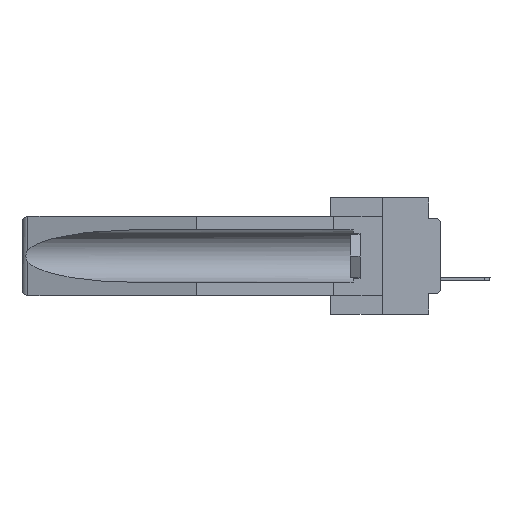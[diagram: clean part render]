
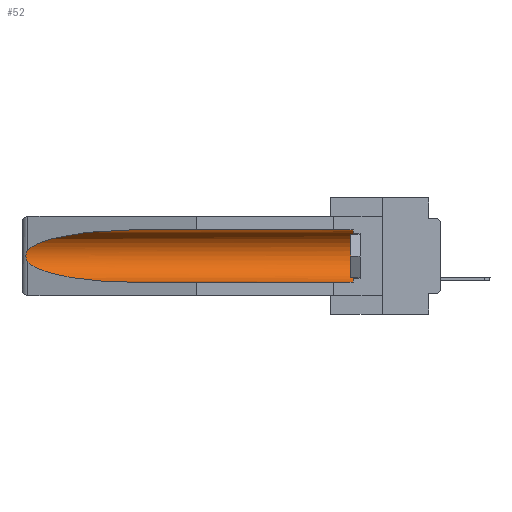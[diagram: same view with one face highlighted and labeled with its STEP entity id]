
A CAD part, left-side view. The second image highlights one B-rep face of the part: STEP entity #52.
In plain terms, the highlighted cylindrical face has radius 2.857 mm (diameter 5.715 mm), a partial arc.
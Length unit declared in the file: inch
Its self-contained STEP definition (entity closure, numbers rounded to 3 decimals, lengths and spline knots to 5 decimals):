
#52 = ADVANCED_FACE ( 'NONE', ( #21755 ), #23921, .F. ) ;
#111 = B_SPLINE_CURVE_WITH_KNOTS ( 'NONE', 3,
 ( #18449, #18297, #6467, #27815, #15988, #25214, #16144, #2009, #18753, #25517 ),
 .UNSPECIFIED., .F., .F.,
 ( 4, 2, 2, 2, 4 ),
 ( 0., 0.00029, 0.00058, 0.00087, 0.00117 ),
 .UNSPECIFIED. ) ;
#756 = VECTOR ( 'NONE', #5604, 39.37008 ) ;
#907 = DIRECTION ( 'NONE',  ( 0., 0., 1. ) ) ;
#1017 = LINE ( 'NONE', #10353, #756 ) ;
#1035 = LINE ( 'NONE', #10519, #4008 ) ;
#1042 = EDGE_CURVE ( 'NONE', #15640, #15206, #111, .T. ) ;
#1517 = CARTESIAN_POINT ( 'NONE',  ( 0.155, 1.07973, -0.059 ) ) ;
#2009 = CARTESIAN_POINT ( 'NONE',  ( 0.26655, 1.53094, -0.18657 ) ) ;
#2273 = VERTEX_POINT ( 'NONE', #16155 ) ;
#4008 = VECTOR ( 'NONE', #27600, 39.37008 ) ;
#4174 = EDGE_CURVE ( 'NONE', #28721, #12093, #25974, .T. ) ;
#4538 =( BOUNDED_CURVE ( )  B_SPLINE_CURVE ( 3, ( #1517, #29317, #10863, #10254 ),
 .UNSPECIFIED., .F., .F. ) 
 B_SPLINE_CURVE_WITH_KNOTS ( ( 4, 4 ),
 ( 4.71239, 6.08839 ),
 .UNSPECIFIED. ) 
 CURVE ( )  GEOMETRIC_REPRESENTATION_ITEM ( )  RATIONAL_B_SPLINE_CURVE ( ( 1., 0.848, 0.848, 1. ) ) 
 REPRESENTATION_ITEM ( '' )  );
#5159 = AXIS2_PLACEMENT_3D ( 'NONE', #24554, #22099, #907 ) ;
#5604 = DIRECTION ( 'NONE',  ( 0., 1., 0. ) ) ;
#5646 = EDGE_CURVE ( 'NONE', #12093, #2273, #1017, .T. ) ;
#6467 = CARTESIAN_POINT ( 'NONE',  ( 0.26654, 1.53092, -0.15636 ) ) ;
#7896 = ORIENTED_EDGE ( 'NONE', *, *, #11293, .T. ) ;
#9016 = AXIS2_PLACEMENT_3D ( 'NONE', #21608, #14836, #9902 ) ;
#9123 = ORIENTED_EDGE ( 'NONE', *, *, #5646, .T. ) ;
#9902 = DIRECTION ( 'NONE',  ( 0., 0., 1. ) ) ;
#10254 = CARTESIAN_POINT ( 'NONE',  ( 0.26537, 1.52718, -0.14972 ) ) ;
#10353 = CARTESIAN_POINT ( 'NONE',  ( 0.155, -0.30754, -0.059 ) ) ;
#10519 = CARTESIAN_POINT ( 'NONE',  ( 0.155, -0.30754, -0.284 ) ) ;
#10863 = CARTESIAN_POINT ( 'NONE',  ( 0.25451, 1.48313, -0.09465 ) ) ;
#10957 = CARTESIAN_POINT ( 'NONE',  ( 0.21114, 1.30732, -0.284 ) ) ;
#11293 = EDGE_CURVE ( 'NONE', #15206, #25546, #17063, .T. ) ;
#12093 = VERTEX_POINT ( 'NONE', #14445 ) ;
#12406 = EDGE_CURVE ( 'NONE', #2273, #15640, #4538, .T. ) ;
#12456 = CARTESIAN_POINT ( 'NONE',  ( 0.155, 0.126, -0.284 ) ) ;
#13138 = CARTESIAN_POINT ( 'NONE',  ( 0.25451, 1.48313, -0.24835 ) ) ;
#13657 = ORIENTED_EDGE ( 'NONE', *, *, #14958, .F. ) ;
#14445 = CARTESIAN_POINT ( 'NONE',  ( 0.155, 0.126, -0.059 ) ) ;
#14836 = DIRECTION ( 'NONE',  ( 0., 1., 0. ) ) ;
#14958 = EDGE_CURVE ( 'NONE', #28721, #25546, #1035, .T. ) ;
#15206 = VERTEX_POINT ( 'NONE', #30043 ) ;
#15640 = VERTEX_POINT ( 'NONE', #30145 ) ;
#15988 = CARTESIAN_POINT ( 'NONE',  ( 0.2675, 1.53308, -0.16763 ) ) ;
#16144 = CARTESIAN_POINT ( 'NONE',  ( 0.2673, 1.53269, -0.17917 ) ) ;
#16155 = CARTESIAN_POINT ( 'NONE',  ( 0.155, 1.07973, -0.059 ) ) ;
#16351 = CARTESIAN_POINT ( 'NONE',  ( 0.155, 1.07973, -0.284 ) ) ;
#17063 =( BOUNDED_CURVE ( )  B_SPLINE_CURVE ( 3, ( #18212, #13138, #10957, #27116 ),
 .UNSPECIFIED., .F., .F. ) 
 B_SPLINE_CURVE_WITH_KNOTS ( ( 4, 4 ),
 ( 0.1948, 1.5708 ),
 .UNSPECIFIED. ) 
 CURVE ( )  GEOMETRIC_REPRESENTATION_ITEM ( )  RATIONAL_B_SPLINE_CURVE ( ( 1., 0.848, 0.848, 1. ) ) 
 REPRESENTATION_ITEM ( '' )  );
#18212 = CARTESIAN_POINT ( 'NONE',  ( 0.26537, 1.52718, -0.19328 ) ) ;
#18297 = CARTESIAN_POINT ( 'NONE',  ( 0.26597, 1.52961, -0.15275 ) ) ;
#18449 = CARTESIAN_POINT ( 'NONE',  ( 0.26537, 1.52718, -0.14972 ) ) ;
#18753 = CARTESIAN_POINT ( 'NONE',  ( 0.26597, 1.5296, -0.19026 ) ) ;
#21608 = CARTESIAN_POINT ( 'NONE',  ( 0.155, -0.30754, -0.1715 ) ) ;
#21755 = FACE_OUTER_BOUND ( 'NONE', #29941, .T. ) ;
#22099 = DIRECTION ( 'NONE',  ( 0., -1., 0. ) ) ;
#23921 = CYLINDRICAL_SURFACE ( 'NONE', #9016, 0.1125 ) ;
#24145 = ORIENTED_EDGE ( 'NONE', *, *, #1042, .T. ) ;
#24554 = CARTESIAN_POINT ( 'NONE',  ( 0.155, 0.126, -0.1715 ) ) ;
#25214 = CARTESIAN_POINT ( 'NONE',  ( 0.2675, 1.53308, -0.17534 ) ) ;
#25517 = CARTESIAN_POINT ( 'NONE',  ( 0.26537, 1.52718, -0.19328 ) ) ;
#25546 = VERTEX_POINT ( 'NONE', #16351 ) ;
#25974 = CIRCLE ( 'NONE', #5159, 0.1125 ) ;
#26927 = ORIENTED_EDGE ( 'NONE', *, *, #12406, .T. ) ;
#27116 = CARTESIAN_POINT ( 'NONE',  ( 0.155, 1.07973, -0.284 ) ) ;
#27600 = DIRECTION ( 'NONE',  ( 0., 1., 0. ) ) ;
#27815 = CARTESIAN_POINT ( 'NONE',  ( 0.2673, 1.5327, -0.16383 ) ) ;
#28721 = VERTEX_POINT ( 'NONE', #12456 ) ;
#28724 = ORIENTED_EDGE ( 'NONE', *, *, #4174, .T. ) ;
#29317 = CARTESIAN_POINT ( 'NONE',  ( 0.21114, 1.30732, -0.059 ) ) ;
#29941 = EDGE_LOOP ( 'NONE', ( #26927, #24145, #7896, #13657, #28724, #9123 ) ) ;
#30043 = CARTESIAN_POINT ( 'NONE',  ( 0.26537, 1.52718, -0.19328 ) ) ;
#30145 = CARTESIAN_POINT ( 'NONE',  ( 0.26537, 1.52718, -0.14972 ) ) ;
